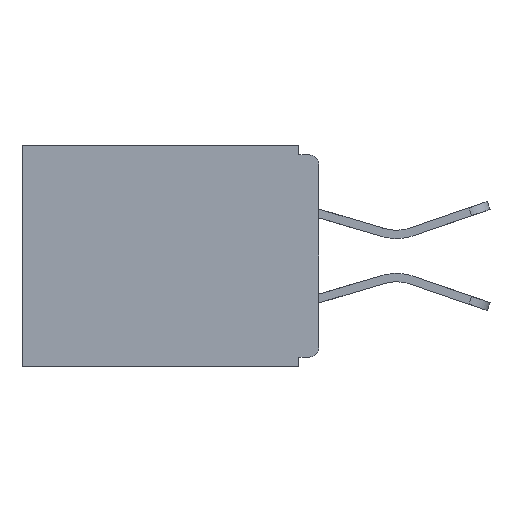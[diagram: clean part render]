
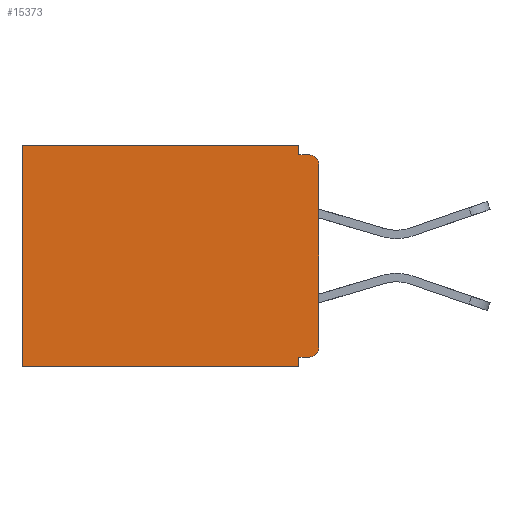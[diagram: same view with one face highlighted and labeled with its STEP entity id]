
A CAD part, left-side view. The second image highlights one B-rep face of the part: STEP entity #15373.
In plain terms, the highlighted planar face has unit normal (-1, 0, 0).
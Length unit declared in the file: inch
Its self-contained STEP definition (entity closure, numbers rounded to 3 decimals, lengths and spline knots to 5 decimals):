
#103 = LINE ( 'NONE', #6383, #11173 ) ;
#239 = CARTESIAN_POINT ( 'NONE',  ( 0.298, 0., -0.328 ) ) ;
#682 = CARTESIAN_POINT ( 'NONE',  ( 0.298, 0., 0. ) ) ;
#696 = DIRECTION ( 'NONE',  ( 0., 0., -1. ) ) ;
#743 = DIRECTION ( 'NONE',  ( 0., 1., 0. ) ) ;
#855 = ORIENTED_EDGE ( 'NONE', *, *, #4897, .F. ) ;
#883 = CARTESIAN_POINT ( 'NONE',  ( 0.298, 0., -0.015 ) ) ;
#949 = LINE ( 'NONE', #682, #13074 ) ;
#1481 = ORIENTED_EDGE ( 'NONE', *, *, #7342, .T. ) ;
#1611 = CARTESIAN_POINT ( 'NONE',  ( 0.298, 0.031, -0.343 ) ) ;
#1669 = EDGE_CURVE ( 'NONE', #15713, #5084, #16531, .T. ) ;
#2246 = ORIENTED_EDGE ( 'NONE', *, *, #16248, .T. ) ;
#2278 = EDGE_CURVE ( 'NONE', #12955, #2737, #103, .T. ) ;
#2636 = LINE ( 'NONE', #6630, #3445 ) ;
#2737 = VERTEX_POINT ( 'NONE', #13792 ) ;
#2934 = AXIS2_PLACEMENT_3D ( 'NONE', #4559, #5920, #696 ) ;
#3166 = CARTESIAN_POINT ( 'NONE',  ( 0.298, 0.031, 0. ) ) ;
#3445 = VECTOR ( 'NONE', #9231, 39.37008 ) ;
#3731 = PLANE ( 'NONE',  #4127 ) ;
#3790 = DIRECTION ( 'NONE',  ( 0., 0., -1. ) ) ;
#3865 = ORIENTED_EDGE ( 'NONE', *, *, #2278, .F. ) ;
#4127 = AXIS2_PLACEMENT_3D ( 'NONE', #11625, #9016, #3790 ) ;
#4217 = DIRECTION ( 'NONE',  ( 0., 1., 0. ) ) ;
#4234 = CARTESIAN_POINT ( 'NONE',  ( 0.298, 0.015, -0.015 ) ) ;
#4327 = CARTESIAN_POINT ( 'NONE',  ( 0.298, 0.031, -0.328 ) ) ;
#4404 = CARTESIAN_POINT ( 'NONE',  ( 0.298, 0.031, -0.015 ) ) ;
#4559 = CARTESIAN_POINT ( 'NONE',  ( 0.298, 0.015, -0.03 ) ) ;
#4837 = VERTEX_POINT ( 'NONE', #9957 ) ;
#4897 = EDGE_CURVE ( 'NONE', #6681, #5084, #9848, .T. ) ;
#5070 = LINE ( 'NONE', #10383, #12927 ) ;
#5084 = VERTEX_POINT ( 'NONE', #4234 ) ;
#5313 = ORIENTED_EDGE ( 'NONE', *, *, #8437, .T. ) ;
#5920 = DIRECTION ( 'NONE',  ( -1., 0., 0. ) ) ;
#6173 = CARTESIAN_POINT ( 'NONE',  ( 0.298, 0.46, 0. ) ) ;
#6322 = DIRECTION ( 'NONE',  ( -1., 0., 0. ) ) ;
#6383 = CARTESIAN_POINT ( 'NONE',  ( 0.298, 0., -0.343 ) ) ;
#6495 = VERTEX_POINT ( 'NONE', #6173 ) ;
#6573 = EDGE_LOOP ( 'NONE', ( #10685, #855, #12615, #1481, #5313, #3865, #15585, #11012, #2246, #7243 ) ) ;
#6630 = CARTESIAN_POINT ( 'NONE',  ( 0.298, 0.46, 0. ) ) ;
#6681 = VERTEX_POINT ( 'NONE', #4404 ) ;
#6804 = EDGE_CURVE ( 'NONE', #14935, #6681, #10006, .T. ) ;
#7243 = ORIENTED_EDGE ( 'NONE', *, *, #8143, .F. ) ;
#7342 = EDGE_CURVE ( 'NONE', #14935, #6495, #949, .T. ) ;
#7964 = CARTESIAN_POINT ( 'NONE',  ( 0.298, 0.015, -0.328 ) ) ;
#8143 = EDGE_CURVE ( 'NONE', #15713, #4837, #5070, .T. ) ;
#8176 = EDGE_CURVE ( 'NONE', #14044, #12955, #16015, .T. ) ;
#8323 = FACE_OUTER_BOUND ( 'NONE', #6573, .T. ) ;
#8423 = VERTEX_POINT ( 'NONE', #7964 ) ;
#8437 = EDGE_CURVE ( 'NONE', #6495, #2737, #2636, .T. ) ;
#8965 = VECTOR ( 'NONE', #13841, 39.37008 ) ;
#8997 = VECTOR ( 'NONE', #9914, 39.37008 ) ;
#9006 = VECTOR ( 'NONE', #15346, 39.37008 ) ;
#9016 = DIRECTION ( 'NONE',  ( 1., 0., 0. ) ) ;
#9231 = DIRECTION ( 'NONE',  ( 0., 0., -1. ) ) ;
#9402 = DIRECTION ( 'NONE',  ( 0., 1., 0. ) ) ;
#9848 = LINE ( 'NONE', #883, #9006 ) ;
#9914 = DIRECTION ( 'NONE',  ( 0., 0., -1. ) ) ;
#9957 = CARTESIAN_POINT ( 'NONE',  ( 0.298, 0., -0.313 ) ) ;
#10006 = LINE ( 'NONE', #12409, #8965 ) ;
#10334 = DIRECTION ( 'NONE',  ( 0., 0., -1. ) ) ;
#10383 = CARTESIAN_POINT ( 'NONE',  ( 0.298, 0., 0. ) ) ;
#10685 = ORIENTED_EDGE ( 'NONE', *, *, #1669, .T. ) ;
#10721 = VECTOR ( 'NONE', #4217, 39.37008 ) ;
#11012 = ORIENTED_EDGE ( 'NONE', *, *, #13510, .F. ) ;
#11173 = VECTOR ( 'NONE', #9402, 39.37008 ) ;
#11625 = CARTESIAN_POINT ( 'NONE',  ( 0.298, 0., 0. ) ) ;
#12409 = CARTESIAN_POINT ( 'NONE',  ( 0.298, 0.031, -0.343 ) ) ;
#12604 = CIRCLE ( 'NONE', #14943, 0.015 ) ;
#12615 = ORIENTED_EDGE ( 'NONE', *, *, #6804, .F. ) ;
#12927 = VECTOR ( 'NONE', #16057, 39.37008 ) ;
#12955 = VERTEX_POINT ( 'NONE', #1611 ) ;
#13074 = VECTOR ( 'NONE', #743, 39.37008 ) ;
#13382 = LINE ( 'NONE', #239, #10721 ) ;
#13510 = EDGE_CURVE ( 'NONE', #8423, #14044, #13382, .T. ) ;
#13792 = CARTESIAN_POINT ( 'NONE',  ( 0.298, 0.46, -0.343 ) ) ;
#13824 = CARTESIAN_POINT ( 'NONE',  ( 0.298, 0.031, -0.343 ) ) ;
#13841 = DIRECTION ( 'NONE',  ( 0., 0., -1. ) ) ;
#14044 = VERTEX_POINT ( 'NONE', #4327 ) ;
#14194 = CARTESIAN_POINT ( 'NONE',  ( 0.298, 0., -0.03 ) ) ;
#14227 = CARTESIAN_POINT ( 'NONE',  ( 0.298, 0.015, -0.313 ) ) ;
#14935 = VERTEX_POINT ( 'NONE', #3166 ) ;
#14943 = AXIS2_PLACEMENT_3D ( 'NONE', #14227, #6322, #10334 ) ;
#15346 = DIRECTION ( 'NONE',  ( 0., -1., 0. ) ) ;
#15373 = ADVANCED_FACE ( 'NONE', ( #8323 ), #3731, .F. ) ;
#15585 = ORIENTED_EDGE ( 'NONE', *, *, #8176, .F. ) ;
#15713 = VERTEX_POINT ( 'NONE', #14194 ) ;
#16015 = LINE ( 'NONE', #13824, #8997 ) ;
#16057 = DIRECTION ( 'NONE',  ( 0., 0., -1. ) ) ;
#16248 = EDGE_CURVE ( 'NONE', #8423, #4837, #12604, .T. ) ;
#16531 = CIRCLE ( 'NONE', #2934, 0.015 ) ;
